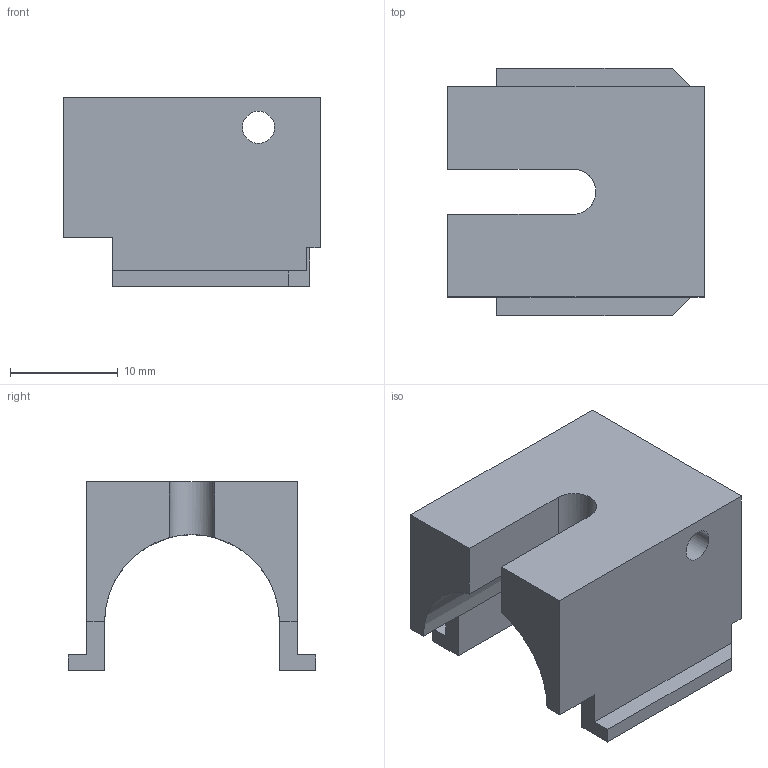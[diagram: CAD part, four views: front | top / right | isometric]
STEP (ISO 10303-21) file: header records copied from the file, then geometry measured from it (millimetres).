
FILE_DESCRIPTION(/* description */ (''),/* implementation_level */ '2;1');
FILE_NAME(/* name */ 'DD19.2 Front Rail.stp',/* time_stamp */ '2021-02-04T13:29:13-06:00',/* author */ ('johne'),/* organization */ (''),/* preprocessor_version */ 'ST-DEVELOPER v18',/* originating_system */ 'Autodesk Inventor 2020',/* authorisation */ '');
FILE_SCHEMA (('AUTOMOTIVE_DESIGN { 1 0 10303 214 3 1 1 }'));
Length unit declared in the file: inch
Products named in the file (1): 19 front rail
Bounding box: 23.86 x 23 x 17.5 mm (x, y, z)
Volume: 3548.8 mm3; surface area: 2753.2 mm2
Topology: 1 solids, 1 shells, 29 faces, 81 edges, 54 vertices
Faces by surface type: plane 26, cylinder 3
Full cylindrical faces by diameter (mm): 3 x1
Entity records: 985 total; most frequent: CARTESIAN_POINT 182, ORIENTED_EDGE 162, DIRECTION 148, EDGE_CURVE 81, LINE 72, VECTOR 72, VERTEX_POINT 54, AXIS2_PLACEMENT_3D 38
